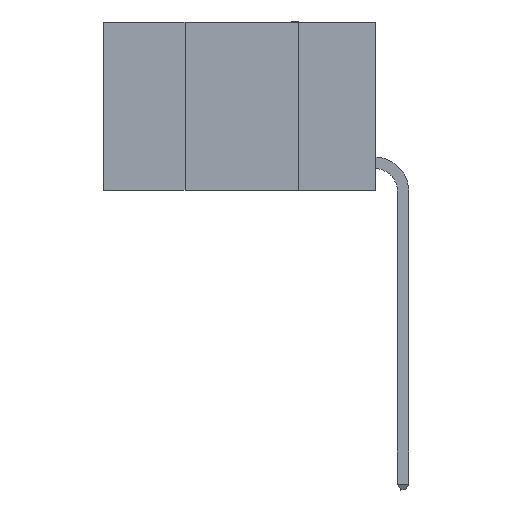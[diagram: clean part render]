
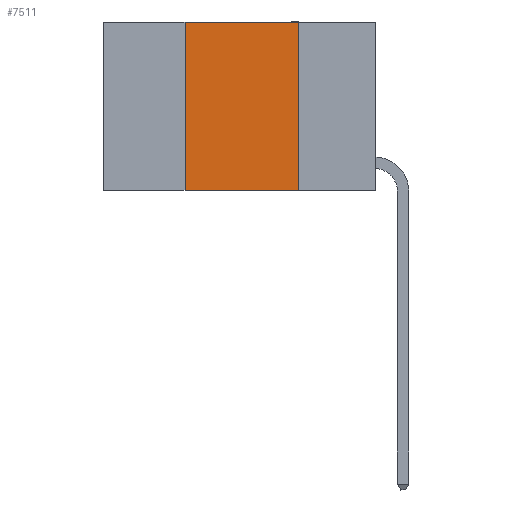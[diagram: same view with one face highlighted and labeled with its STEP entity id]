
A CAD part, left-side view. The second image highlights one B-rep face of the part: STEP entity #7511.
In plain terms, the highlighted planar face has unit normal (-1, 0, 0).
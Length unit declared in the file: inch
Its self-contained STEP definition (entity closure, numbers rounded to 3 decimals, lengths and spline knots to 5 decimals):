
#518 = DIRECTION ( 'NONE',  ( 0., 0., 1. ) ) ;
#1882 = DIRECTION ( 'NONE',  ( 0., 0., -1. ) ) ;
#2317 = EDGE_CURVE ( 'NONE', #26850, #23143, #18845, .T. ) ;
#3358 = VECTOR ( 'NONE', #6882, 39.37008 ) ;
#4038 = ORIENTED_EDGE ( 'NONE', *, *, #28457, .T. ) ;
#4665 = VECTOR ( 'NONE', #1882, 39.37008 ) ;
#4773 = VECTOR ( 'NONE', #518, 39.37008 ) ;
#5728 = CARTESIAN_POINT ( 'NONE',  ( 0., 0.6, -0.37 ) ) ;
#6816 = CARTESIAN_POINT ( 'NONE',  ( 0., 0.42, 0. ) ) ;
#6882 = DIRECTION ( 'NONE',  ( 0., -1., 0. ) ) ;
#7511 = ADVANCED_FACE ( 'NONE', ( #17602 ), #22231, .F. ) ;
#8003 = EDGE_CURVE ( 'NONE', #23143, #14138, #25389, .T. ) ;
#8368 = LINE ( 'NONE', #5728, #27013 ) ;
#10843 = ORIENTED_EDGE ( 'NONE', *, *, #2317, .F. ) ;
#13139 = DIRECTION ( 'NONE',  ( 0., 0., -1. ) ) ;
#14138 = VERTEX_POINT ( 'NONE', #20806 ) ;
#15295 = DIRECTION ( 'NONE',  ( 1., 0., 0. ) ) ;
#15861 = CARTESIAN_POINT ( 'NONE',  ( 0., 0.17, 0. ) ) ;
#17253 = EDGE_CURVE ( 'NONE', #22526, #26850, #29303, .T. ) ;
#17602 = FACE_OUTER_BOUND ( 'NONE', #27711, .T. ) ;
#17965 = DIRECTION ( 'NONE',  ( 0., -1., 0. ) ) ;
#18688 = CARTESIAN_POINT ( 'NONE',  ( 0., 0.6, 0. ) ) ;
#18845 = LINE ( 'NONE', #18688, #3358 ) ;
#19548 = ORIENTED_EDGE ( 'NONE', *, *, #17253, .F. ) ;
#20376 = CARTESIAN_POINT ( 'NONE',  ( 0., 0.6, 0. ) ) ;
#20806 = CARTESIAN_POINT ( 'NONE',  ( 0., 0.17, -0.37 ) ) ;
#22231 = PLANE ( 'NONE',  #25228 ) ;
#22526 = VERTEX_POINT ( 'NONE', #26433 ) ;
#23143 = VERTEX_POINT ( 'NONE', #26551 ) ;
#24129 = ORIENTED_EDGE ( 'NONE', *, *, #8003, .F. ) ;
#24508 = CARTESIAN_POINT ( 'NONE',  ( 0., 0.42, 0. ) ) ;
#25228 = AXIS2_PLACEMENT_3D ( 'NONE', #20376, #15295, #13139 ) ;
#25389 = LINE ( 'NONE', #15861, #4665 ) ;
#26433 = CARTESIAN_POINT ( 'NONE',  ( 0., 0.42, -0.37 ) ) ;
#26551 = CARTESIAN_POINT ( 'NONE',  ( 0., 0.17, 0. ) ) ;
#26850 = VERTEX_POINT ( 'NONE', #6816 ) ;
#27013 = VECTOR ( 'NONE', #17965, 39.37008 ) ;
#27711 = EDGE_LOOP ( 'NONE', ( #24129, #10843, #19548, #4038 ) ) ;
#28457 = EDGE_CURVE ( 'NONE', #22526, #14138, #8368, .T. ) ;
#29303 = LINE ( 'NONE', #24508, #4773 ) ;
